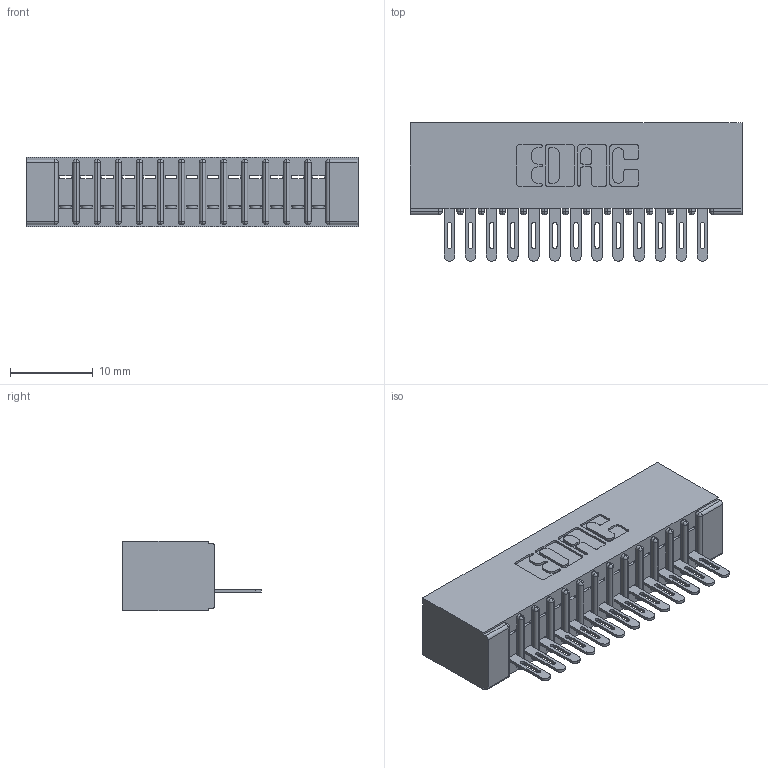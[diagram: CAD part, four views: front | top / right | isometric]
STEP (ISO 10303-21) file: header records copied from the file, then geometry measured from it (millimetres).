
FILE_DESCRIPTION (( 'STEP AP203' ), '1' );
FILE_NAME ('341-013-500-101.STEP', '2018-08-06T03:44:10', ( '' ), ( '' ), 'SwSTEP 2.0', 'SolidWorks 2016', '' );
FILE_SCHEMA (( 'CONFIG_CONTROL_DESIGN' ));
Length unit declared in the file: inch
Products named in the file (3): 341-292-001_341-292-100; 341-013-500-101; 341 Part_No Mounting Lugs
Assembly tree (14 placements, depth 2):
  341-013-500-101
    341 Part_No Mounting Lugs
    341-292-001_341-292-100  x13
Bounding box: 40.01 x 16.69 x 8.38 mm (x, y, z)
Volume: 2354.7 mm3; surface area: 4510.8 mm2
Topology: 14 solids, 14 shells, 1174 faces, 3373 edges, 2166 vertices
Faces by surface type: plane 701, cylinder 421, sphere 28, torus 24
Entity records: 18910 total; most frequent: CARTESIAN_POINT 3198, ORIENTED_EDGE 3186, DIRECTION 3113, EDGE_CURVE 1593, VECTOR 1255, LINE 1255, VERTEX_POINT 1014, AXIS2_PLACEMENT_3D 929
